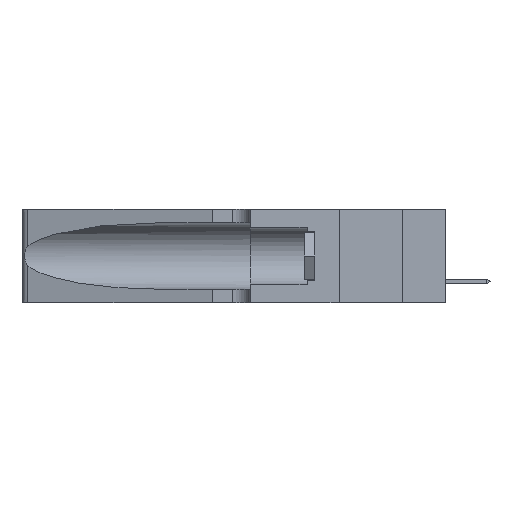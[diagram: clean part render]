
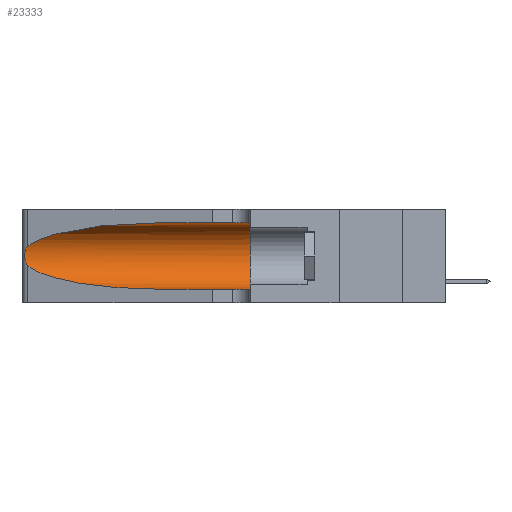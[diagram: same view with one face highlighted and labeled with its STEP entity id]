
A CAD part, left-side view. The second image highlights one B-rep face of the part: STEP entity #23333.
In plain terms, the highlighted cylindrical face has radius 3.308 mm (diameter 6.617 mm), a partial arc.
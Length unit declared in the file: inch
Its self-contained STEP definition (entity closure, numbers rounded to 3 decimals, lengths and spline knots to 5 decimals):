
#625 = LINE ( 'NONE', #6003, #23175 ) ;
#925 = EDGE_CURVE ( 'NONE', #16392, #29039, #12123, .T. ) ;
#1165 = DIRECTION ( 'NONE',  ( 0., -1., 0. ) ) ;
#2352 = EDGE_CURVE ( 'NONE', #26180, #17587, #625, .T. ) ;
#2485 = ORIENTED_EDGE ( 'NONE', *, *, #30538, .T. ) ;
#2938 = ORIENTED_EDGE ( 'NONE', *, *, #28903, .T. ) ;
#2978 = CARTESIAN_POINT ( 'NONE',  ( 0.1305, 1.61858, 0.185 ) ) ;
#3574 = CARTESIAN_POINT ( 'NONE',  ( 0.25555, 1.22993, 0.14849 ) ) ;
#3892 = B_SPLINE_CURVE_WITH_KNOTS ( 'NONE', 3,
 ( #27571, #7532, #12620, #9654, #15589, #28352, #5653, #30550, #15354, #5881, #23697, #11061, #3574, #13747 ),
 .UNSPECIFIED., .F., .F.,
 ( 4, 2, 2, 2, 2, 2, 4 ),
 ( 0., 0.00027, 0.00053, 0.00107, 0.0016, 0.00187, 0.00214 ),
 .UNSPECIFIED. ) ;
#4175 = CARTESIAN_POINT ( 'NONE',  ( 0.18966, 0.96281, 0.31525 ) ) ;
#4791 = ORIENTED_EDGE ( 'NONE', *, *, #925, .F. ) ;
#5653 = CARTESIAN_POINT ( 'NONE',  ( 0.26075, 1.23896, 0.19203 ) ) ;
#5881 = CARTESIAN_POINT ( 'NONE',  ( 0.25856, 1.23593, 0.16098 ) ) ;
#6003 = CARTESIAN_POINT ( 'NONE',  ( 0.1305, 1.61858, 0.05475 ) ) ;
#6227 = CARTESIAN_POINT ( 'NONE',  ( 0.25487, 1.22718, 0.14631 ) ) ;
#6607 = EDGE_CURVE ( 'NONE', #24214, #12220, #3892, .T. ) ;
#6897 = CARTESIAN_POINT ( 'NONE',  ( 0.18966, 0.96281, 0.05475 ) ) ;
#7532 = CARTESIAN_POINT ( 'NONE',  ( 0.25555, 1.22994, 0.2215 ) ) ;
#7946 = ORIENTED_EDGE ( 'NONE', *, *, #6607, .T. ) ;
#8615 = AXIS2_PLACEMENT_3D ( 'NONE', #21011, #31288, #26184 ) ;
#8847 = DIRECTION ( 'NONE',  ( 0., 0., -1. ) ) ;
#8962 = VECTOR ( 'NONE', #31868, 39.37008 ) ;
#9382 = EDGE_LOOP ( 'NONE', ( #2485, #7946, #2938, #15914, #28654, #4791 ) ) ;
#9390 = CIRCLE ( 'NONE', #8615, 0.13025 ) ;
#9654 = CARTESIAN_POINT ( 'NONE',  ( 0.25787, 1.23484, 0.2124 ) ) ;
#10220 = CARTESIAN_POINT ( 'NONE',  ( 0.1305, 0.72297, 0.31525 ) ) ;
#11061 = CARTESIAN_POINT ( 'NONE',  ( 0.25639, 1.23186, 0.15144 ) ) ;
#11192 = CARTESIAN_POINT ( 'NONE',  ( 0.1305, 0.35, 0.31525 ) ) ;
#11988 = CARTESIAN_POINT ( 'NONE',  ( 0.2373, 1.15595, 0.28018 ) ) ;
#12123 = LINE ( 'NONE', #19567, #8962 ) ;
#12220 = VERTEX_POINT ( 'NONE', #21768 ) ;
#12620 = CARTESIAN_POINT ( 'NONE',  ( 0.25639, 1.23184, 0.21858 ) ) ;
#13747 = CARTESIAN_POINT ( 'NONE',  ( 0.25487, 1.22718, 0.14631 ) ) ;
#14361 =( BOUNDED_CURVE ( )  B_SPLINE_CURVE ( 3, ( #6227, #29603, #6897, #24496 ),
 .UNSPECIFIED., .F., .T. ) 
 B_SPLINE_CURVE_WITH_KNOTS ( ( 4, 4 ),
 ( 3.44316, 4.71239 ),
 .UNSPECIFIED. ) 
 CURVE ( )  GEOMETRIC_REPRESENTATION_ITEM ( )  RATIONAL_B_SPLINE_CURVE ( ( 1., 0.87, 0.87, 1. ) ) 
 REPRESENTATION_ITEM ( '' )  );
#15354 = CARTESIAN_POINT ( 'NONE',  ( 0.26017, 1.23833, 0.17102 ) ) ;
#15589 = CARTESIAN_POINT ( 'NONE',  ( 0.25854, 1.2359, 0.20912 ) ) ;
#15914 = ORIENTED_EDGE ( 'NONE', *, *, #2352, .T. ) ;
#16392 = VERTEX_POINT ( 'NONE', #10220 ) ;
#17587 = VERTEX_POINT ( 'NONE', #32364 ) ;
#18147 = CARTESIAN_POINT ( 'NONE',  ( 0.1305, 0.72297, 0.05475 ) ) ;
#18361 = DIRECTION ( 'NONE',  ( 0., -1., 0. ) ) ;
#19567 = CARTESIAN_POINT ( 'NONE',  ( 0.1305, 1.61858, 0.31525 ) ) ;
#21011 = CARTESIAN_POINT ( 'NONE',  ( 0.1305, 0.35, 0.185 ) ) ;
#21219 = CYLINDRICAL_SURFACE ( 'NONE', #32186, 0.13025 ) ;
#21768 = CARTESIAN_POINT ( 'NONE',  ( 0.25487, 1.22718, 0.14631 ) ) ;
#21873 = CARTESIAN_POINT ( 'NONE',  ( 0.25487, 1.22718, 0.22369 ) ) ;
#22123 = EDGE_CURVE ( 'NONE', #29039, #17587, #9390, .T. ) ;
#22301 = CARTESIAN_POINT ( 'NONE',  ( 0.25487, 1.22718, 0.22369 ) ) ;
#22664 =( BOUNDED_CURVE ( )  B_SPLINE_CURVE ( 3, ( #24410, #4175, #11988, #21873 ),
 .UNSPECIFIED., .F., .F. ) 
 B_SPLINE_CURVE_WITH_KNOTS ( ( 4, 4 ),
 ( 1.5708, 2.84003 ),
 .UNSPECIFIED. ) 
 CURVE ( )  GEOMETRIC_REPRESENTATION_ITEM ( )  RATIONAL_B_SPLINE_CURVE ( ( 1., 0.87, 0.87, 1. ) ) 
 REPRESENTATION_ITEM ( '' )  );
#23175 = VECTOR ( 'NONE', #1165, 39.37008 ) ;
#23333 = ADVANCED_FACE ( 'NONE', ( #31526 ), #21219, .F. ) ;
#23697 = CARTESIAN_POINT ( 'NONE',  ( 0.25789, 1.23486, 0.15765 ) ) ;
#24214 = VERTEX_POINT ( 'NONE', #22301 ) ;
#24410 = CARTESIAN_POINT ( 'NONE',  ( 0.1305, 0.72297, 0.31525 ) ) ;
#24496 = CARTESIAN_POINT ( 'NONE',  ( 0.1305, 0.72297, 0.05475 ) ) ;
#26180 = VERTEX_POINT ( 'NONE', #18147 ) ;
#26184 = DIRECTION ( 'NONE',  ( 0., 0., 1. ) ) ;
#27571 = CARTESIAN_POINT ( 'NONE',  ( 0.25487, 1.22718, 0.22369 ) ) ;
#28352 = CARTESIAN_POINT ( 'NONE',  ( 0.26018, 1.23835, 0.19895 ) ) ;
#28654 = ORIENTED_EDGE ( 'NONE', *, *, #22123, .F. ) ;
#28903 = EDGE_CURVE ( 'NONE', #12220, #26180, #14361, .T. ) ;
#29039 = VERTEX_POINT ( 'NONE', #11192 ) ;
#29603 = CARTESIAN_POINT ( 'NONE',  ( 0.2373, 1.15595, 0.08982 ) ) ;
#30538 = EDGE_CURVE ( 'NONE', #16392, #24214, #22664, .T. ) ;
#30550 = CARTESIAN_POINT ( 'NONE',  ( 0.26075, 1.23896, 0.178 ) ) ;
#31288 = DIRECTION ( 'NONE',  ( 0., 1., 0. ) ) ;
#31526 = FACE_OUTER_BOUND ( 'NONE', #9382, .T. ) ;
#31868 = DIRECTION ( 'NONE',  ( 0., -1., 0. ) ) ;
#32186 = AXIS2_PLACEMENT_3D ( 'NONE', #2978, #18361, #8847 ) ;
#32364 = CARTESIAN_POINT ( 'NONE',  ( 0.1305, 0.35, 0.05475 ) ) ;
